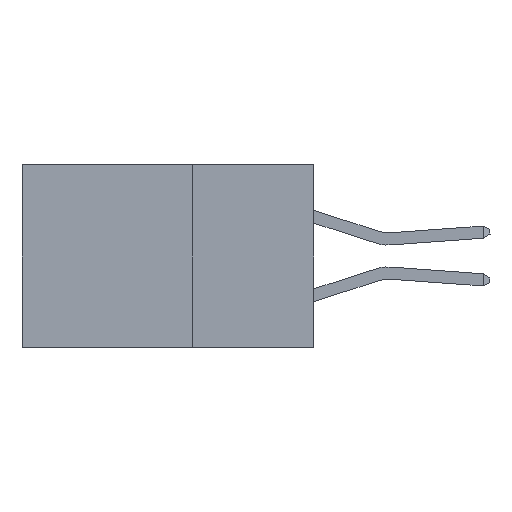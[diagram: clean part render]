
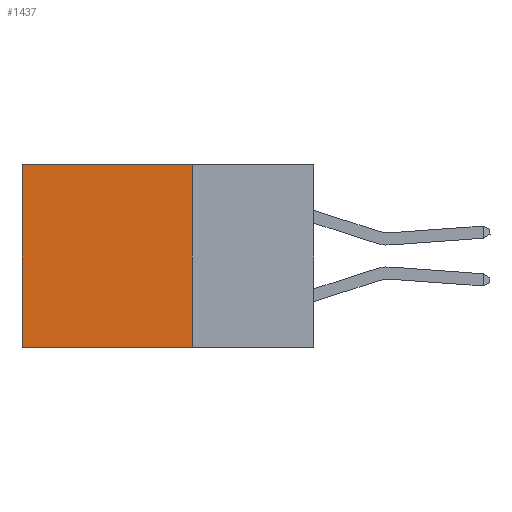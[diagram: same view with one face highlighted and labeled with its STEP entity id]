
A CAD part, left-side view. The second image highlights one B-rep face of the part: STEP entity #1437.
In plain terms, the highlighted planar face has unit normal (-1, 0, 0).
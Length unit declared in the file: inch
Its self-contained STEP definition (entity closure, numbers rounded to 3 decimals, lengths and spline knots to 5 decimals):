
#49 = VERTEX_POINT ( 'NONE', #1093 ) ;
#477 = CARTESIAN_POINT ( 'NONE',  ( 0.2875, 0.25, -0.375 ) ) ;
#719 = VECTOR ( 'NONE', #1124, 39.37008 ) ;
#1093 = CARTESIAN_POINT ( 'NONE',  ( 0.2875, 0.6, -0.375 ) ) ;
#1124 = DIRECTION ( 'NONE',  ( 0., 0., -1. ) ) ;
#1437 = ADVANCED_FACE ( 'NONE', ( #3337 ), #9079, .F. ) ;
#1619 = LINE ( 'NONE', #10627, #4290 ) ;
#1759 = DIRECTION ( 'NONE',  ( 0., 0., -1. ) ) ;
#1973 = CARTESIAN_POINT ( 'NONE',  ( 0.2875, 0.6, 0. ) ) ;
#2475 = ORIENTED_EDGE ( 'NONE', *, *, #8422, .T. ) ;
#3337 = FACE_OUTER_BOUND ( 'NONE', #16681, .T. ) ;
#3901 = DIRECTION ( 'NONE',  ( 1., 0., 0. ) ) ;
#4290 = VECTOR ( 'NONE', #6553, 39.37008 ) ;
#4831 = LINE ( 'NONE', #9736, #15703 ) ;
#4933 = VERTEX_POINT ( 'NONE', #477 ) ;
#6342 = VECTOR ( 'NONE', #16900, 39.37008 ) ;
#6553 = DIRECTION ( 'NONE',  ( 0., 1., 0. ) ) ;
#6962 = LINE ( 'NONE', #15587, #6342 ) ;
#7217 = ORIENTED_EDGE ( 'NONE', *, *, #14768, .T. ) ;
#7628 = VERTEX_POINT ( 'NONE', #11691 ) ;
#8422 = EDGE_CURVE ( 'NONE', #9522, #49, #15097, .T. ) ;
#8991 = ORIENTED_EDGE ( 'NONE', *, *, #11497, .F. ) ;
#9079 = PLANE ( 'NONE',  #17002 ) ;
#9522 = VERTEX_POINT ( 'NONE', #1973 ) ;
#9736 = CARTESIAN_POINT ( 'NONE',  ( 0.2875, 0.25, -0.375 ) ) ;
#10595 = ORIENTED_EDGE ( 'NONE', *, *, #14853, .F. ) ;
#10627 = CARTESIAN_POINT ( 'NONE',  ( 0.2875, 0.25, -0.375 ) ) ;
#11497 = EDGE_CURVE ( 'NONE', #7628, #4933, #4831, .T. ) ;
#11610 = CARTESIAN_POINT ( 'NONE',  ( 0.2875, 0.6, -0.375 ) ) ;
#11691 = CARTESIAN_POINT ( 'NONE',  ( 0.2875, 0.25, 0. ) ) ;
#13078 = CARTESIAN_POINT ( 'NONE',  ( 0.2875, 0.25, -0.375 ) ) ;
#14409 = DIRECTION ( 'NONE',  ( 0., 0., -1. ) ) ;
#14768 = EDGE_CURVE ( 'NONE', #7628, #9522, #6962, .T. ) ;
#14853 = EDGE_CURVE ( 'NONE', #4933, #49, #1619, .T. ) ;
#15097 = LINE ( 'NONE', #11610, #719 ) ;
#15587 = CARTESIAN_POINT ( 'NONE',  ( 0.2875, 0.25, 0. ) ) ;
#15703 = VECTOR ( 'NONE', #1759, 39.37008 ) ;
#16681 = EDGE_LOOP ( 'NONE', ( #2475, #10595, #8991, #7217 ) ) ;
#16900 = DIRECTION ( 'NONE',  ( 0., 1., 0. ) ) ;
#17002 = AXIS2_PLACEMENT_3D ( 'NONE', #13078, #3901, #14409 ) ;
